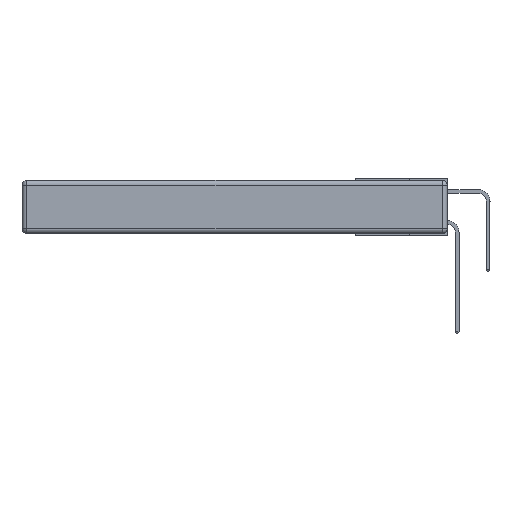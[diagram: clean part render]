
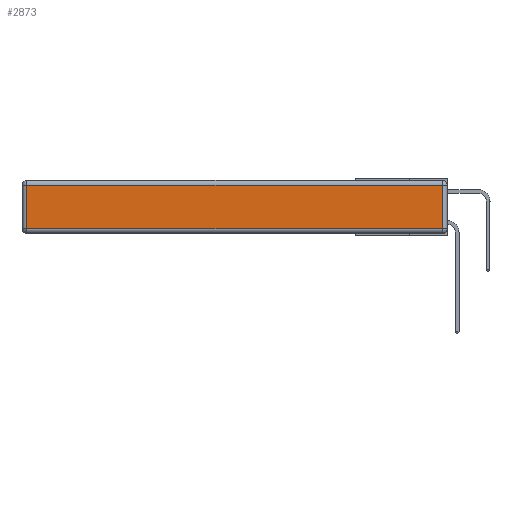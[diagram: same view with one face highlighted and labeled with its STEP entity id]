
A CAD part, left-side view. The second image highlights one B-rep face of the part: STEP entity #2873.
In plain terms, the highlighted planar face has unit normal (-1, 0, 0).
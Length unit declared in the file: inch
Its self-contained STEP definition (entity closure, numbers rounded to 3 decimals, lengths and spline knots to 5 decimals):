
#663 = EDGE_CURVE ( 'NONE', #14234, #16637, #11672, .T. ) ;
#1908 = CARTESIAN_POINT ( 'NONE',  ( 0., 0., -0.313 ) ) ;
#2376 = AXIS2_PLACEMENT_3D ( 'NONE', #7919, #6530, #3784 ) ;
#2841 = ORIENTED_EDGE ( 'NONE', *, *, #663, .T. ) ;
#2873 = ADVANCED_FACE ( 'NONE', ( #11524 ), #13645, .T. ) ;
#3001 = CARTESIAN_POINT ( 'NONE',  ( 0., 2.72, -0.313 ) ) ;
#3750 = CARTESIAN_POINT ( 'NONE',  ( 0., 2.72, -0.03 ) ) ;
#3784 = DIRECTION ( 'NONE',  ( 0., 0., 1. ) ) ;
#4147 = DIRECTION ( 'NONE',  ( 0., 1., 0. ) ) ;
#5284 = EDGE_CURVE ( 'NONE', #17791, #5722, #13634, .T. ) ;
#5360 = ORIENTED_EDGE ( 'NONE', *, *, #5284, .T. ) ;
#5722 = VERTEX_POINT ( 'NONE', #16731 ) ;
#6487 = VECTOR ( 'NONE', #4147, 39.37008 ) ;
#6530 = DIRECTION ( 'NONE',  ( -1., 0., 0. ) ) ;
#6796 = VECTOR ( 'NONE', #17509, 39.37008 ) ;
#7363 = CARTESIAN_POINT ( 'NONE',  ( 0., 0.03, -0.343 ) ) ;
#7919 = CARTESIAN_POINT ( 'NONE',  ( 0., 0., -0.343 ) ) ;
#8097 = EDGE_CURVE ( 'NONE', #5722, #14234, #12950, .T. ) ;
#8457 = CARTESIAN_POINT ( 'NONE',  ( 0., 0.03, -0.313 ) ) ;
#8527 = VECTOR ( 'NONE', #9932, 39.37008 ) ;
#9932 = DIRECTION ( 'NONE',  ( 0., 0., 1. ) ) ;
#10617 = LINE ( 'NONE', #1908, #6796 ) ;
#10758 = EDGE_CURVE ( 'NONE', #16637, #17791, #10617, .T. ) ;
#11524 = FACE_OUTER_BOUND ( 'NONE', #18175, .T. ) ;
#11672 = LINE ( 'NONE', #14830, #12750 ) ;
#12750 = VECTOR ( 'NONE', #17666, 39.37008 ) ;
#12950 = LINE ( 'NONE', #17000, #6487 ) ;
#13634 = LINE ( 'NONE', #7363, #8527 ) ;
#13645 = PLANE ( 'NONE',  #2376 ) ;
#14234 = VERTEX_POINT ( 'NONE', #3750 ) ;
#14525 = ORIENTED_EDGE ( 'NONE', *, *, #10758, .T. ) ;
#14830 = CARTESIAN_POINT ( 'NONE',  ( 0., 2.72, -0.343 ) ) ;
#16637 = VERTEX_POINT ( 'NONE', #3001 ) ;
#16731 = CARTESIAN_POINT ( 'NONE',  ( 0., 0.03, -0.03 ) ) ;
#16905 = ORIENTED_EDGE ( 'NONE', *, *, #8097, .T. ) ;
#17000 = CARTESIAN_POINT ( 'NONE',  ( 0., 2.75, -0.03 ) ) ;
#17509 = DIRECTION ( 'NONE',  ( 0., -1., 0. ) ) ;
#17666 = DIRECTION ( 'NONE',  ( 0., 0., -1. ) ) ;
#17791 = VERTEX_POINT ( 'NONE', #8457 ) ;
#18175 = EDGE_LOOP ( 'NONE', ( #14525, #5360, #16905, #2841 ) ) ;
